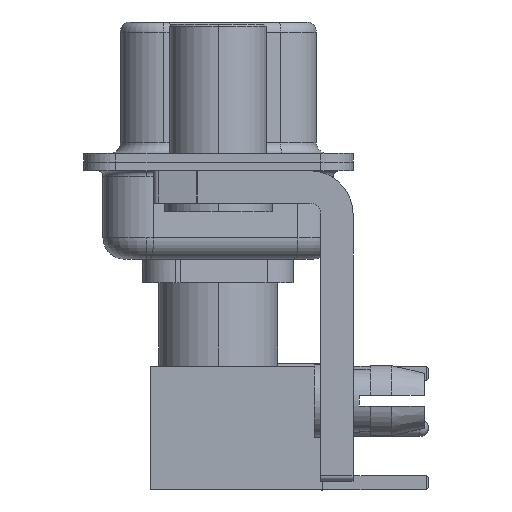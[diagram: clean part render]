
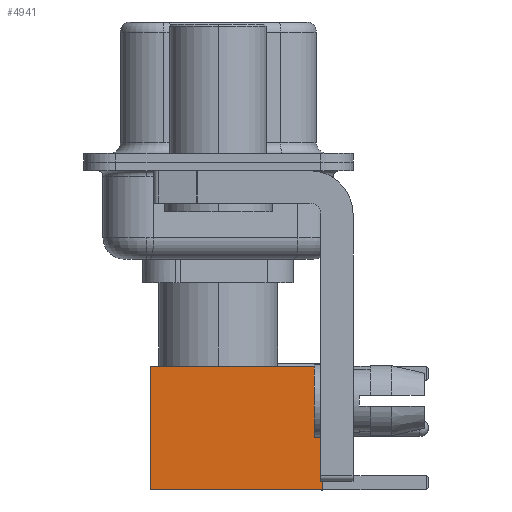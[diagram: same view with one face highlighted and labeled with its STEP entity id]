
A CAD part, left-side view. The second image highlights one B-rep face of the part: STEP entity #4941.
In plain terms, the highlighted face is planar.
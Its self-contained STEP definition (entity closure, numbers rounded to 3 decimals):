
#1369 = EDGE_LOOP ( 'NONE', ( #2029, #5839, #13942, #12303 ) ) ;
#1644 = PLANE ( 'NONE',  #23120 ) ;
#2029 = ORIENTED_EDGE ( 'NONE', *, *, #28661, .T. ) ;
#2360 = CARTESIAN_POINT ( 'NONE',  ( 0., 2.875, 0. ) ) ;
#2519 = CARTESIAN_POINT ( 'NONE',  ( 0., 2.875, 8. ) ) ;
#3707 = CARTESIAN_POINT ( 'NONE',  ( -2.875, 2.875, 0. ) ) ;
#4548 = LINE ( 'NONE', #2360, #20563 ) ;
#4941 = ADVANCED_FACE ( 'NONE', ( #13387 ), #1644, .T. ) ;
#5839 = ORIENTED_EDGE ( 'NONE', *, *, #10185, .T. ) ;
#7038 = LINE ( 'NONE', #2519, #27363 ) ;
#7258 = VERTEX_POINT ( 'NONE', #23779 ) ;
#7277 = VERTEX_POINT ( 'NONE', #28453 ) ;
#8523 = CARTESIAN_POINT ( 'NONE',  ( 2.875, 2.875, 0. ) ) ;
#8879 = CARTESIAN_POINT ( 'NONE',  ( 2.875, 2.875, 0. ) ) ;
#9864 = VECTOR ( 'NONE', #18423, 1000. ) ;
#10185 = EDGE_CURVE ( 'NONE', #7277, #15663, #4548, .T. ) ;
#12303 = ORIENTED_EDGE ( 'NONE', *, *, #29563, .F. ) ;
#12820 = VECTOR ( 'NONE', #20904, 1000. ) ;
#13387 = FACE_OUTER_BOUND ( 'NONE', #1369, .T. ) ;
#13942 = ORIENTED_EDGE ( 'NONE', *, *, #18373, .F. ) ;
#15663 = VERTEX_POINT ( 'NONE', #23478 ) ;
#18373 = EDGE_CURVE ( 'NONE', #29192, #15663, #27606, .T. ) ;
#18423 = DIRECTION ( 'NONE',  ( 0., 0., -1. ) ) ;
#19620 = CARTESIAN_POINT ( 'NONE',  ( -2.875, 2.875, 8. ) ) ;
#20563 = VECTOR ( 'NONE', #28441, 1000. ) ;
#20904 = DIRECTION ( 'NONE',  ( 0., 0., -1. ) ) ;
#23120 = AXIS2_PLACEMENT_3D ( 'NONE', #8523, #25250, #30102 ) ;
#23478 = CARTESIAN_POINT ( 'NONE',  ( -2.875, 2.875, 0. ) ) ;
#23779 = CARTESIAN_POINT ( 'NONE',  ( 2.875, 2.875, 8. ) ) ;
#25250 = DIRECTION ( 'NONE',  ( 0., 1., 0. ) ) ;
#26101 = DIRECTION ( 'NONE',  ( -1., 0., 0. ) ) ;
#27363 = VECTOR ( 'NONE', #26101, 1000. ) ;
#27606 = LINE ( 'NONE', #3707, #12820 ) ;
#28441 = DIRECTION ( 'NONE',  ( -1., 0., 0. ) ) ;
#28453 = CARTESIAN_POINT ( 'NONE',  ( 2.875, 2.875, 0. ) ) ;
#28661 = EDGE_CURVE ( 'NONE', #7258, #7277, #30304, .T. ) ;
#29192 = VERTEX_POINT ( 'NONE', #19620 ) ;
#29563 = EDGE_CURVE ( 'NONE', #7258, #29192, #7038, .T. ) ;
#30102 = DIRECTION ( 'NONE',  ( 0., 0., 1. ) ) ;
#30304 = LINE ( 'NONE', #8879, #9864 ) ;
